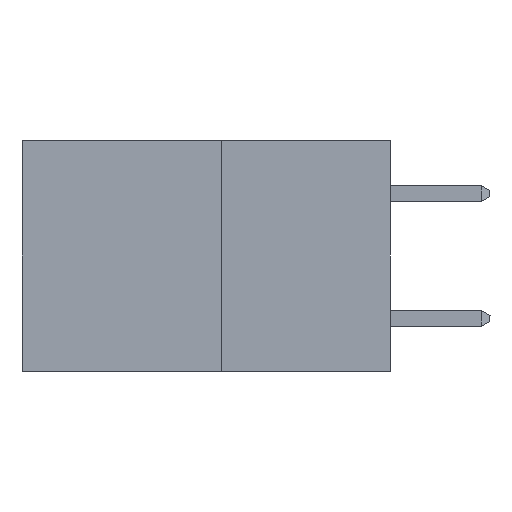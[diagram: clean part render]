
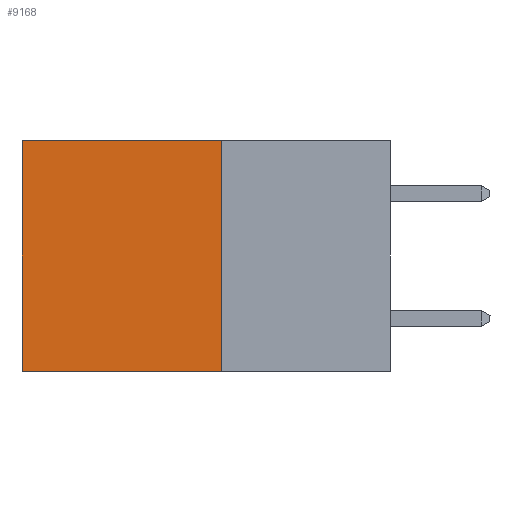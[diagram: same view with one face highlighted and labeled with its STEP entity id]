
A CAD part, left-side view. The second image highlights one B-rep face of the part: STEP entity #9168.
In plain terms, the highlighted planar face has unit normal (-1, 0, 0).
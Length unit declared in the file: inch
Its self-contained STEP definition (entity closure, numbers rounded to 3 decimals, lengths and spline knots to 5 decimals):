
#144 = EDGE_CURVE ( 'NONE', #3985, #1578, #7913, .T. ) ;
#610 = CARTESIAN_POINT ( 'NONE',  ( 0.277, 0.27, 0. ) ) ;
#644 = CARTESIAN_POINT ( 'NONE',  ( 0.277, 0.59, 0. ) ) ;
#684 = ORIENTED_EDGE ( 'NONE', *, *, #1898, .T. ) ;
#1140 = ORIENTED_EDGE ( 'NONE', *, *, #144, .F. ) ;
#1291 = CARTESIAN_POINT ( 'NONE',  ( 0.277, 0.59, -0.37 ) ) ;
#1578 = VERTEX_POINT ( 'NONE', #7144 ) ;
#1830 = EDGE_CURVE ( 'NONE', #1578, #9839, #9703, .T. ) ;
#1898 = EDGE_CURVE ( 'NONE', #4722, #9839, #4861, .T. ) ;
#2366 = EDGE_CURVE ( 'NONE', #3985, #4722, #3677, .T. ) ;
#2564 = AXIS2_PLACEMENT_3D ( 'NONE', #7763, #10975, #6118 ) ;
#2824 = ORIENTED_EDGE ( 'NONE', *, *, #2366, .T. ) ;
#2917 = CARTESIAN_POINT ( 'NONE',  ( 0.277, 0.27, -0.37 ) ) ;
#3427 = VECTOR ( 'NONE', #5816, 39.37008 ) ;
#3677 = LINE ( 'NONE', #610, #3427 ) ;
#3985 = VERTEX_POINT ( 'NONE', #10026 ) ;
#4722 = VERTEX_POINT ( 'NONE', #644 ) ;
#4739 = DIRECTION ( 'NONE',  ( 0., 0., -1. ) ) ;
#4861 = LINE ( 'NONE', #1291, #6552 ) ;
#5696 = VECTOR ( 'NONE', #9923, 39.37008 ) ;
#5816 = DIRECTION ( 'NONE',  ( 0., 1., 0. ) ) ;
#6118 = DIRECTION ( 'NONE',  ( 0., 0., -1. ) ) ;
#6552 = VECTOR ( 'NONE', #4739, 39.37008 ) ;
#7144 = CARTESIAN_POINT ( 'NONE',  ( 0.277, 0.27, -0.37 ) ) ;
#7591 = VECTOR ( 'NONE', #9493, 39.37008 ) ;
#7763 = CARTESIAN_POINT ( 'NONE',  ( 0.277, 0.27, -0.37 ) ) ;
#7913 = LINE ( 'NONE', #10762, #5696 ) ;
#8684 = EDGE_LOOP ( 'NONE', ( #684, #9205, #1140, #2824 ) ) ;
#9138 = CARTESIAN_POINT ( 'NONE',  ( 0.277, 0.59, -0.37 ) ) ;
#9168 = ADVANCED_FACE ( 'NONE', ( #10205 ), #9352, .F. ) ;
#9205 = ORIENTED_EDGE ( 'NONE', *, *, #1830, .F. ) ;
#9352 = PLANE ( 'NONE',  #2564 ) ;
#9493 = DIRECTION ( 'NONE',  ( 0., 1., 0. ) ) ;
#9703 = LINE ( 'NONE', #2917, #7591 ) ;
#9839 = VERTEX_POINT ( 'NONE', #9138 ) ;
#9923 = DIRECTION ( 'NONE',  ( 0., 0., -1. ) ) ;
#10026 = CARTESIAN_POINT ( 'NONE',  ( 0.277, 0.27, 0. ) ) ;
#10205 = FACE_OUTER_BOUND ( 'NONE', #8684, .T. ) ;
#10762 = CARTESIAN_POINT ( 'NONE',  ( 0.277, 0.27, -0.37 ) ) ;
#10975 = DIRECTION ( 'NONE',  ( 1., 0., 0. ) ) ;
